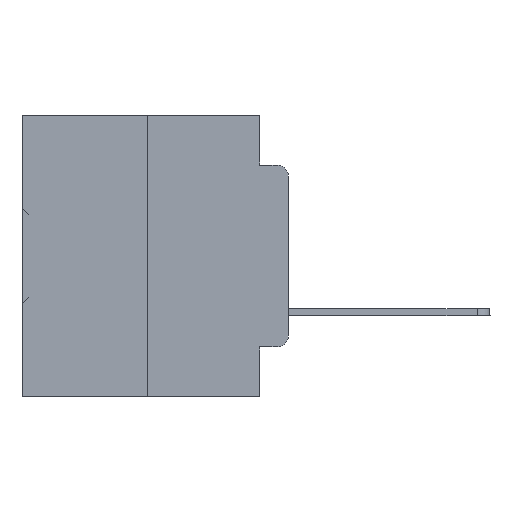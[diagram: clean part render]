
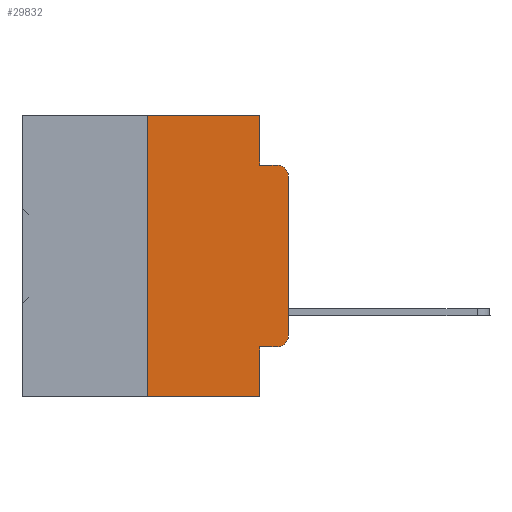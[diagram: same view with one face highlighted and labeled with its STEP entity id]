
A CAD part, left-side view. The second image highlights one B-rep face of the part: STEP entity #29832.
In plain terms, the highlighted planar face has unit normal (-1, 0, 0).
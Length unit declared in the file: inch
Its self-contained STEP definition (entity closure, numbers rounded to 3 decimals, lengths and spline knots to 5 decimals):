
#94 = CARTESIAN_POINT ( 'NONE',  ( 0., 0.25, 0. ) ) ;
#295 = DIRECTION ( 'NONE',  ( 0., 0., 1. ) ) ;
#703 = EDGE_CURVE ( 'NONE', #8197, #16176, #3784, .T. ) ;
#2485 = LINE ( 'NONE', #32886, #11171 ) ;
#2715 = VERTEX_POINT ( 'NONE', #24007 ) ;
#2755 = AXIS2_PLACEMENT_3D ( 'NONE', #32453, #6227, #3422 ) ;
#3422 = DIRECTION ( 'NONE',  ( 0., 0., -1. ) ) ;
#3476 = FACE_OUTER_BOUND ( 'NONE', #7725, .T. ) ;
#3784 = LINE ( 'NONE', #31680, #37212 ) ;
#3818 = LINE ( 'NONE', #30800, #17159 ) ;
#4051 = CARTESIAN_POINT ( 'NONE',  ( 0., 0.02, -0.0885 ) ) ;
#4113 = AXIS2_PLACEMENT_3D ( 'NONE', #20142, #17920, #23745 ) ;
#4160 = CARTESIAN_POINT ( 'NONE',  ( 0., 0., -0.3915 ) ) ;
#4655 = EDGE_CURVE ( 'NONE', #14609, #29726, #9919, .T. ) ;
#5047 = EDGE_CURVE ( 'NONE', #19221, #8197, #3818, .T. ) ;
#6227 = DIRECTION ( 'NONE',  ( -1., 0., 0. ) ) ;
#6276 = ORIENTED_EDGE ( 'NONE', *, *, #4655, .T. ) ;
#7185 = VECTOR ( 'NONE', #295, 39.37008 ) ;
#7526 = DIRECTION ( 'NONE',  ( 0., 0., 1. ) ) ;
#7725 = EDGE_LOOP ( 'NONE', ( #6276, #18395, #33800, #31301, #26563, #35815, #15486, #11808, #9717, #37657 ) ) ;
#7893 = CARTESIAN_POINT ( 'NONE',  ( 0., 0.051, -0.4115 ) ) ;
#8197 = VERTEX_POINT ( 'NONE', #94 ) ;
#8353 = EDGE_CURVE ( 'NONE', #31365, #29527, #27325, .T. ) ;
#8736 = DIRECTION ( 'NONE',  ( 0., 0., -1. ) ) ;
#9717 = ORIENTED_EDGE ( 'NONE', *, *, #8353, .T. ) ;
#9919 = LINE ( 'NONE', #32391, #7185 ) ;
#10154 = CARTESIAN_POINT ( 'NONE',  ( 0., 0.051, 0. ) ) ;
#11171 = VECTOR ( 'NONE', #15416, 39.37008 ) ;
#11324 = DIRECTION ( 'NONE',  ( -1., 0., 0. ) ) ;
#11714 = EDGE_CURVE ( 'NONE', #29527, #14609, #28637, .T. ) ;
#11808 = ORIENTED_EDGE ( 'NONE', *, *, #31408, .F. ) ;
#13086 = CARTESIAN_POINT ( 'NONE',  ( 0., 0.25, -0.5 ) ) ;
#13354 = EDGE_CURVE ( 'NONE', #29726, #21038, #14415, .T. ) ;
#13652 = VERTEX_POINT ( 'NONE', #16292 ) ;
#14415 = CIRCLE ( 'NONE', #2755, 0.02 ) ;
#14609 = VERTEX_POINT ( 'NONE', #4160 ) ;
#15416 = DIRECTION ( 'NONE',  ( 0., 0., -1. ) ) ;
#15486 = ORIENTED_EDGE ( 'NONE', *, *, #36745, .T. ) ;
#16176 = VERTEX_POINT ( 'NONE', #10154 ) ;
#16292 = CARTESIAN_POINT ( 'NONE',  ( 0., 0.051, -0.0885 ) ) ;
#17159 = VECTOR ( 'NONE', #7526, 39.37008 ) ;
#17581 = LINE ( 'NONE', #32692, #34483 ) ;
#17920 = DIRECTION ( 'NONE',  ( 1., 0., 0. ) ) ;
#18177 = DIRECTION ( 'NONE',  ( 0., -1., 0. ) ) ;
#18395 = ORIENTED_EDGE ( 'NONE', *, *, #13354, .T. ) ;
#18767 = DIRECTION ( 'NONE',  ( 0., -1., 0. ) ) ;
#19221 = VERTEX_POINT ( 'NONE', #13086 ) ;
#20142 = CARTESIAN_POINT ( 'NONE',  ( 0., 0.473, 0. ) ) ;
#21038 = VERTEX_POINT ( 'NONE', #4051 ) ;
#21052 = CARTESIAN_POINT ( 'NONE',  ( 0., 0.051, -0.4115 ) ) ;
#21868 = AXIS2_PLACEMENT_3D ( 'NONE', #25762, #11324, #8736 ) ;
#21929 = CARTESIAN_POINT ( 'NONE',  ( 0., 0.051, 0. ) ) ;
#22757 = DIRECTION ( 'NONE',  ( 0., -1., 0. ) ) ;
#23209 = EDGE_CURVE ( 'NONE', #13652, #21038, #36262, .T. ) ;
#23649 = VECTOR ( 'NONE', #24089, 39.37008 ) ;
#23745 = DIRECTION ( 'NONE',  ( 0., 0., -1. ) ) ;
#24007 = CARTESIAN_POINT ( 'NONE',  ( 0., 0.051, -0.5 ) ) ;
#24089 = DIRECTION ( 'NONE',  ( 0., -1., 0. ) ) ;
#24715 = DIRECTION ( 'NONE',  ( 0., 0., -1. ) ) ;
#24783 = VECTOR ( 'NONE', #24715, 39.37008 ) ;
#25762 = CARTESIAN_POINT ( 'NONE',  ( 0., 0.02, -0.3915 ) ) ;
#26563 = ORIENTED_EDGE ( 'NONE', *, *, #703, .F. ) ;
#27325 = LINE ( 'NONE', #21052, #23649 ) ;
#28637 = CIRCLE ( 'NONE', #21868, 0.02 ) ;
#28871 = EDGE_CURVE ( 'NONE', #16176, #13652, #32529, .T. ) ;
#29527 = VERTEX_POINT ( 'NONE', #32930 ) ;
#29726 = VERTEX_POINT ( 'NONE', #30434 ) ;
#29832 = ADVANCED_FACE ( 'NONE', ( #3476 ), #31741, .F. ) ;
#30434 = CARTESIAN_POINT ( 'NONE',  ( 0., 0., -0.1085 ) ) ;
#30800 = CARTESIAN_POINT ( 'NONE',  ( 0., 0.25, 0. ) ) ;
#31301 = ORIENTED_EDGE ( 'NONE', *, *, #28871, .F. ) ;
#31365 = VERTEX_POINT ( 'NONE', #7893 ) ;
#31408 = EDGE_CURVE ( 'NONE', #31365, #2715, #2485, .T. ) ;
#31680 = CARTESIAN_POINT ( 'NONE',  ( 0., 0.473, 0. ) ) ;
#31741 = PLANE ( 'NONE',  #4113 ) ;
#32391 = CARTESIAN_POINT ( 'NONE',  ( 0., 0., 0. ) ) ;
#32453 = CARTESIAN_POINT ( 'NONE',  ( 0., 0.02, -0.1085 ) ) ;
#32529 = LINE ( 'NONE', #21929, #24783 ) ;
#32574 = VECTOR ( 'NONE', #18767, 39.37008 ) ;
#32692 = CARTESIAN_POINT ( 'NONE',  ( 0., 0.473, -0.5 ) ) ;
#32886 = CARTESIAN_POINT ( 'NONE',  ( 0., 0.051, 0. ) ) ;
#32930 = CARTESIAN_POINT ( 'NONE',  ( 0., 0.02, -0.4115 ) ) ;
#33690 = CARTESIAN_POINT ( 'NONE',  ( 0., 0.051, -0.0885 ) ) ;
#33800 = ORIENTED_EDGE ( 'NONE', *, *, #23209, .F. ) ;
#34483 = VECTOR ( 'NONE', #18177, 39.37008 ) ;
#35815 = ORIENTED_EDGE ( 'NONE', *, *, #5047, .F. ) ;
#36262 = LINE ( 'NONE', #33690, #32574 ) ;
#36745 = EDGE_CURVE ( 'NONE', #19221, #2715, #17581, .T. ) ;
#37212 = VECTOR ( 'NONE', #22757, 39.37008 ) ;
#37657 = ORIENTED_EDGE ( 'NONE', *, *, #11714, .T. ) ;
